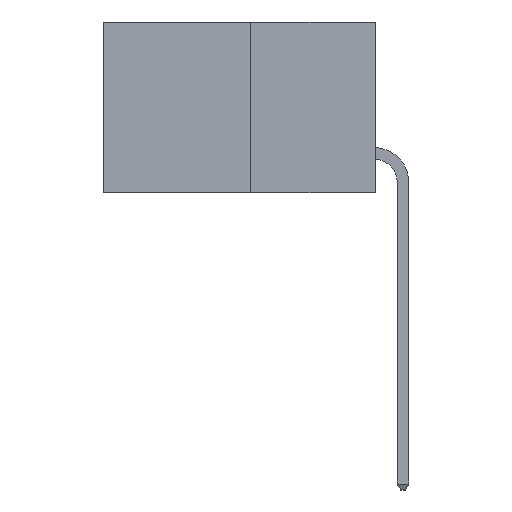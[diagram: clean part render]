
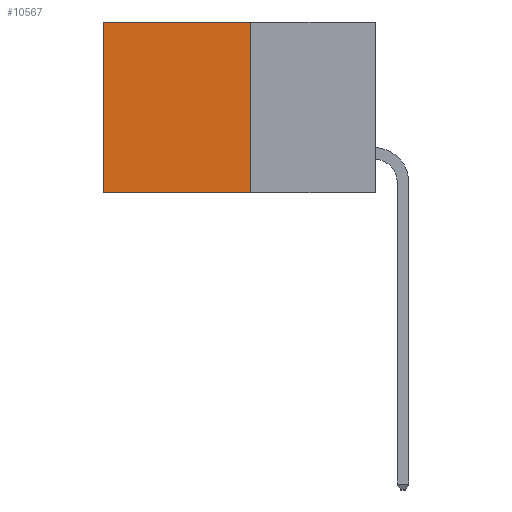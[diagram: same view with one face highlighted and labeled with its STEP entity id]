
A CAD part, left-side view. The second image highlights one B-rep face of the part: STEP entity #10567.
In plain terms, the highlighted planar face has unit normal (-1, 0, 0).
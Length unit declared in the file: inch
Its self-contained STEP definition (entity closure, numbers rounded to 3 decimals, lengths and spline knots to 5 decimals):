
#443 = CARTESIAN_POINT ( 'NONE',  ( 0.277, 0.27, -0.37 ) ) ;
#866 = EDGE_CURVE ( 'NONE', #1290, #7255, #7430, .T. ) ;
#1290 = VERTEX_POINT ( 'NONE', #2015 ) ;
#1803 = CARTESIAN_POINT ( 'NONE',  ( 0.277, 0.27, -0.37 ) ) ;
#2015 = CARTESIAN_POINT ( 'NONE',  ( 0.277, 0.27, 0. ) ) ;
#3418 = ORIENTED_EDGE ( 'NONE', *, *, #866, .T. ) ;
#4294 = DIRECTION ( 'NONE',  ( 1., 0., 0. ) ) ;
#5013 = ORIENTED_EDGE ( 'NONE', *, *, #19999, .F. ) ;
#5395 = DIRECTION ( 'NONE',  ( 0., 1., 0. ) ) ;
#5746 = VECTOR ( 'NONE', #15318, 39.37008 ) ;
#6224 = AXIS2_PLACEMENT_3D ( 'NONE', #17817, #4294, #16179 ) ;
#6329 = LINE ( 'NONE', #1803, #19320 ) ;
#6482 = CARTESIAN_POINT ( 'NONE',  ( 0.277, 0.59, 0. ) ) ;
#6724 = LINE ( 'NONE', #443, #9603 ) ;
#6874 = CARTESIAN_POINT ( 'NONE',  ( 0.277, 0.59, -0.37 ) ) ;
#7255 = VERTEX_POINT ( 'NONE', #6482 ) ;
#7316 = DIRECTION ( 'NONE',  ( 0., 0., -1. ) ) ;
#7430 = LINE ( 'NONE', #12446, #15910 ) ;
#8842 = VERTEX_POINT ( 'NONE', #11625 ) ;
#9603 = VECTOR ( 'NONE', #7316, 39.37008 ) ;
#10567 = ADVANCED_FACE ( 'NONE', ( #18263 ), #14463, .F. ) ;
#11625 = CARTESIAN_POINT ( 'NONE',  ( 0.277, 0.27, -0.37 ) ) ;
#12446 = CARTESIAN_POINT ( 'NONE',  ( 0.277, 0.27, 0. ) ) ;
#12791 = ORIENTED_EDGE ( 'NONE', *, *, #16011, .F. ) ;
#13709 = DIRECTION ( 'NONE',  ( 0., 1., 0. ) ) ;
#14124 = EDGE_LOOP ( 'NONE', ( #15330, #5013, #12791, #3418 ) ) ;
#14463 = PLANE ( 'NONE',  #6224 ) ;
#15318 = DIRECTION ( 'NONE',  ( 0., 0., -1. ) ) ;
#15330 = ORIENTED_EDGE ( 'NONE', *, *, #21826, .T. ) ;
#15910 = VECTOR ( 'NONE', #5395, 39.37008 ) ;
#16011 = EDGE_CURVE ( 'NONE', #1290, #8842, #6724, .T. ) ;
#16179 = DIRECTION ( 'NONE',  ( 0., 0., -1. ) ) ;
#17016 = VERTEX_POINT ( 'NONE', #19061 ) ;
#17817 = CARTESIAN_POINT ( 'NONE',  ( 0.277, 0.27, -0.37 ) ) ;
#18263 = FACE_OUTER_BOUND ( 'NONE', #14124, .T. ) ;
#19061 = CARTESIAN_POINT ( 'NONE',  ( 0.277, 0.59, -0.37 ) ) ;
#19285 = LINE ( 'NONE', #6874, #5746 ) ;
#19320 = VECTOR ( 'NONE', #13709, 39.37008 ) ;
#19999 = EDGE_CURVE ( 'NONE', #8842, #17016, #6329, .T. ) ;
#21826 = EDGE_CURVE ( 'NONE', #7255, #17016, #19285, .T. ) ;
